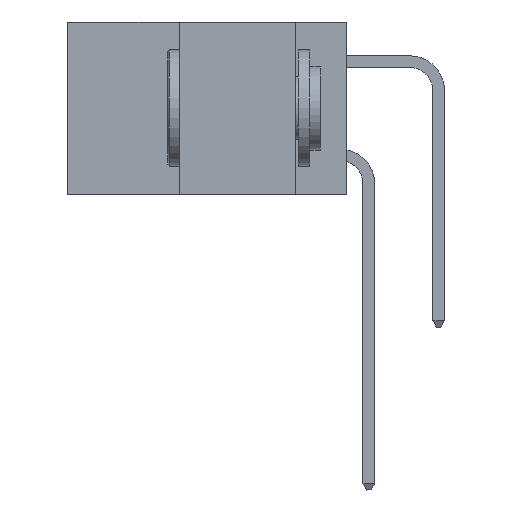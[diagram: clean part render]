
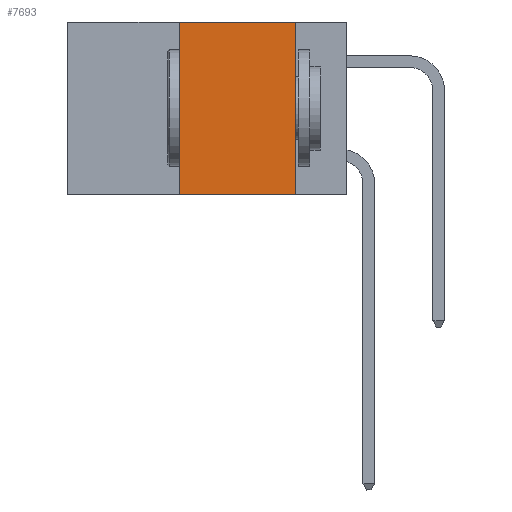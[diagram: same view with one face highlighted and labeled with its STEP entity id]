
A CAD part, left-side view. The second image highlights one B-rep face of the part: STEP entity #7693.
In plain terms, the highlighted planar face has unit normal (-1, 0, 0).
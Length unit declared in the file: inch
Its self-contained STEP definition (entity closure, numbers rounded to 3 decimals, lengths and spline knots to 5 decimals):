
#882 = DIRECTION ( 'NONE',  ( 0., -1., 0. ) ) ;
#3055 = EDGE_CURVE ( 'NONE', #14040, #16645, #5388, .T. ) ;
#5137 = EDGE_CURVE ( 'NONE', #34414, #14040, #31548, .T. ) ;
#5388 = LINE ( 'NONE', #33395, #20848 ) ;
#7693 = ADVANCED_FACE ( 'NONE', ( #8883 ), #33019, .F. ) ;
#8624 = VECTOR ( 'NONE', #15512, 39.37008 ) ;
#8883 = FACE_OUTER_BOUND ( 'NONE', #17797, .T. ) ;
#10119 = VERTEX_POINT ( 'NONE', #23566 ) ;
#10220 = CARTESIAN_POINT ( 'NONE',  ( 0., 0.11, 0. ) ) ;
#12506 = CARTESIAN_POINT ( 'NONE',  ( 0., 0.11, 0. ) ) ;
#13071 = LINE ( 'NONE', #18446, #13991 ) ;
#13170 = DIRECTION ( 'NONE',  ( 0., 0., -1. ) ) ;
#13991 = VECTOR ( 'NONE', #882, 39.37008 ) ;
#14040 = VERTEX_POINT ( 'NONE', #17130 ) ;
#14940 = EDGE_CURVE ( 'NONE', #34414, #10119, #13071, .T. ) ;
#15512 = DIRECTION ( 'NONE',  ( 0., 0., 1. ) ) ;
#15923 = DIRECTION ( 'NONE',  ( 1., 0., 0. ) ) ;
#16645 = VERTEX_POINT ( 'NONE', #12506 ) ;
#17130 = CARTESIAN_POINT ( 'NONE',  ( 0., 0.36, 0. ) ) ;
#17797 = EDGE_LOOP ( 'NONE', ( #18026, #36713, #26989, #22131 ) ) ;
#18026 = ORIENTED_EDGE ( 'NONE', *, *, #32869, .F. ) ;
#18446 = CARTESIAN_POINT ( 'NONE',  ( 0., 0.6, -0.37 ) ) ;
#18549 = VECTOR ( 'NONE', #13170, 39.37008 ) ;
#20848 = VECTOR ( 'NONE', #36218, 39.37008 ) ;
#22131 = ORIENTED_EDGE ( 'NONE', *, *, #14940, .T. ) ;
#23566 = CARTESIAN_POINT ( 'NONE',  ( 0., 0.11, -0.37 ) ) ;
#26127 = LINE ( 'NONE', #10220, #18549 ) ;
#26887 = CARTESIAN_POINT ( 'NONE',  ( 0., 0.36, 0. ) ) ;
#26989 = ORIENTED_EDGE ( 'NONE', *, *, #5137, .F. ) ;
#27099 = CARTESIAN_POINT ( 'NONE',  ( 0., 0.36, -0.37 ) ) ;
#30175 = CARTESIAN_POINT ( 'NONE',  ( 0., 0.6, 0. ) ) ;
#31548 = LINE ( 'NONE', #26887, #8624 ) ;
#32869 = EDGE_CURVE ( 'NONE', #16645, #10119, #26127, .T. ) ;
#33019 = PLANE ( 'NONE',  #34592 ) ;
#33395 = CARTESIAN_POINT ( 'NONE',  ( 0., 0.6, 0. ) ) ;
#34414 = VERTEX_POINT ( 'NONE', #27099 ) ;
#34592 = AXIS2_PLACEMENT_3D ( 'NONE', #30175, #15923, #35837 ) ;
#35837 = DIRECTION ( 'NONE',  ( 0., 0., -1. ) ) ;
#36218 = DIRECTION ( 'NONE',  ( 0., -1., 0. ) ) ;
#36713 = ORIENTED_EDGE ( 'NONE', *, *, #3055, .F. ) ;
